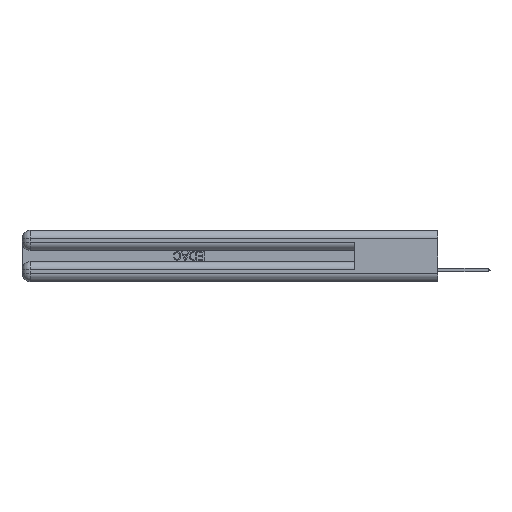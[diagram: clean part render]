
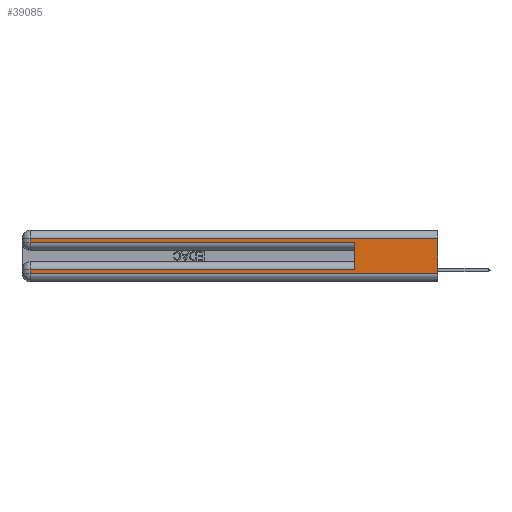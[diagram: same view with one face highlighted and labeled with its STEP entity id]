
A CAD part, left-side view. The second image highlights one B-rep face of the part: STEP entity #39085.
In plain terms, the highlighted planar face has unit normal (-1, 0, 0).
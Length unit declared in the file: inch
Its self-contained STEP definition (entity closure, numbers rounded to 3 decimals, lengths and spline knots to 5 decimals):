
#1454 = CARTESIAN_POINT ( 'NONE',  ( 0., 0., 0.37 ) ) ;
#1602 = VECTOR ( 'NONE', #25481, 39.37008 ) ;
#2188 = VERTEX_POINT ( 'NONE', #9679 ) ;
#2295 = DIRECTION ( 'NONE',  ( 0., -1., 0. ) ) ;
#2531 = EDGE_CURVE ( 'NONE', #8296, #48635, #44984, .T. ) ;
#3287 = LINE ( 'NONE', #25847, #29746 ) ;
#5423 = CARTESIAN_POINT ( 'NONE',  ( 0., 0., 0.37 ) ) ;
#6042 = EDGE_CURVE ( 'NONE', #35684, #14626, #7430, .T. ) ;
#6059 = VERTEX_POINT ( 'NONE', #44478 ) ;
#6721 = DIRECTION ( 'NONE',  ( 0., 0., 1. ) ) ;
#6917 = ORIENTED_EDGE ( 'NONE', *, *, #2531, .T. ) ;
#7396 = ORIENTED_EDGE ( 'NONE', *, *, #19312, .T. ) ;
#7430 = LINE ( 'NONE', #36332, #41964 ) ;
#8296 = VERTEX_POINT ( 'NONE', #38085 ) ;
#9076 = ORIENTED_EDGE ( 'NONE', *, *, #6042, .T. ) ;
#9236 = ORIENTED_EDGE ( 'NONE', *, *, #10892, .T. ) ;
#9393 = DIRECTION ( 'NONE',  ( 1., 0., 0. ) ) ;
#9551 = PLANE ( 'NONE',  #38165 ) ;
#9679 = CARTESIAN_POINT ( 'NONE',  ( 0., 0., 0.31 ) ) ;
#10472 = VECTOR ( 'NONE', #28211, 39.37008 ) ;
#10549 = VECTOR ( 'NONE', #40689, 39.37008 ) ;
#10892 = EDGE_CURVE ( 'NONE', #48635, #6059, #3287, .T. ) ;
#11815 = VERTEX_POINT ( 'NONE', #44315 ) ;
#13110 = CARTESIAN_POINT ( 'NONE',  ( 0., 2.94, 0.37 ) ) ;
#14626 = VERTEX_POINT ( 'NONE', #40916 ) ;
#15193 = LINE ( 'NONE', #13110, #1602 ) ;
#16018 = CARTESIAN_POINT ( 'NONE',  ( 0., 2.94, 0.37 ) ) ;
#17751 = CARTESIAN_POINT ( 'NONE',  ( 0., 0.6, 0.085 ) ) ;
#17789 = LINE ( 'NONE', #32989, #18443 ) ;
#18432 = DIRECTION ( 'NONE',  ( 0., 1., 0. ) ) ;
#18443 = VECTOR ( 'NONE', #44916, 39.37008 ) ;
#18458 = LINE ( 'NONE', #34402, #25841 ) ;
#18507 = ORIENTED_EDGE ( 'NONE', *, *, #33160, .T. ) ;
#19312 = EDGE_CURVE ( 'NONE', #41869, #8296, #17789, .T. ) ;
#21128 = DIRECTION ( 'NONE',  ( 0., 0., -1. ) ) ;
#22199 = CARTESIAN_POINT ( 'NONE',  ( 0., 0., 0.31 ) ) ;
#22242 = VECTOR ( 'NONE', #18432, 39.37008 ) ;
#23038 = CARTESIAN_POINT ( 'NONE',  ( 0., 2.94, 0.285 ) ) ;
#25481 = DIRECTION ( 'NONE',  ( 0., 0., -1. ) ) ;
#25841 = VECTOR ( 'NONE', #6721, 39.37008 ) ;
#25847 = CARTESIAN_POINT ( 'NONE',  ( 0., 0., 0.06 ) ) ;
#26524 = ORIENTED_EDGE ( 'NONE', *, *, #47763, .F. ) ;
#27948 = ORIENTED_EDGE ( 'NONE', *, *, #39744, .F. ) ;
#28211 = DIRECTION ( 'NONE',  ( 0., 0., -1. ) ) ;
#28595 = DIRECTION ( 'NONE',  ( 0., -1., 0. ) ) ;
#29634 = LINE ( 'NONE', #22199, #22242 ) ;
#29657 = LINE ( 'NONE', #1454, #10549 ) ;
#29746 = VECTOR ( 'NONE', #2295, 39.37008 ) ;
#32989 = CARTESIAN_POINT ( 'NONE',  ( 0., 0., 0.085 ) ) ;
#33160 = EDGE_CURVE ( 'NONE', #11815, #35684, #15193, .T. ) ;
#34402 = CARTESIAN_POINT ( 'NONE',  ( 0., 0.6, 0.145 ) ) ;
#34621 = FACE_OUTER_BOUND ( 'NONE', #49822, .T. ) ;
#35614 = ORIENTED_EDGE ( 'NONE', *, *, #35637, .T. ) ;
#35637 = EDGE_CURVE ( 'NONE', #2188, #11815, #29634, .T. ) ;
#35684 = VERTEX_POINT ( 'NONE', #23038 ) ;
#36332 = CARTESIAN_POINT ( 'NONE',  ( 0., 0., 0.285 ) ) ;
#38085 = CARTESIAN_POINT ( 'NONE',  ( 0., 2.94, 0.085 ) ) ;
#38165 = AXIS2_PLACEMENT_3D ( 'NONE', #5423, #9393, #21128 ) ;
#39085 = ADVANCED_FACE ( 'NONE', ( #34621 ), #9551, .F. ) ;
#39744 = EDGE_CURVE ( 'NONE', #2188, #6059, #29657, .T. ) ;
#40689 = DIRECTION ( 'NONE',  ( 0., 0., -1. ) ) ;
#40916 = CARTESIAN_POINT ( 'NONE',  ( 0., 0.6, 0.285 ) ) ;
#41869 = VERTEX_POINT ( 'NONE', #17751 ) ;
#41964 = VECTOR ( 'NONE', #28595, 39.37008 ) ;
#44315 = CARTESIAN_POINT ( 'NONE',  ( 0., 2.94, 0.31 ) ) ;
#44478 = CARTESIAN_POINT ( 'NONE',  ( 0., 0., 0.06 ) ) ;
#44916 = DIRECTION ( 'NONE',  ( 0., 1., 0. ) ) ;
#44984 = LINE ( 'NONE', #16018, #10472 ) ;
#47264 = CARTESIAN_POINT ( 'NONE',  ( 0., 2.94, 0.06 ) ) ;
#47763 = EDGE_CURVE ( 'NONE', #41869, #14626, #18458, .T. ) ;
#48635 = VERTEX_POINT ( 'NONE', #47264 ) ;
#49822 = EDGE_LOOP ( 'NONE', ( #27948, #35614, #18507, #9076, #26524, #7396, #6917, #9236 ) ) ;
